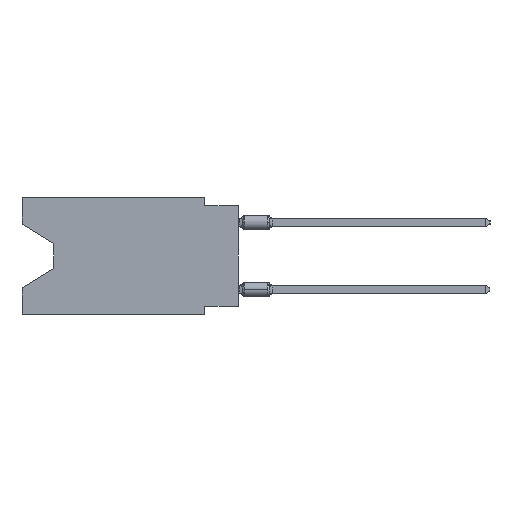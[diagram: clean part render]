
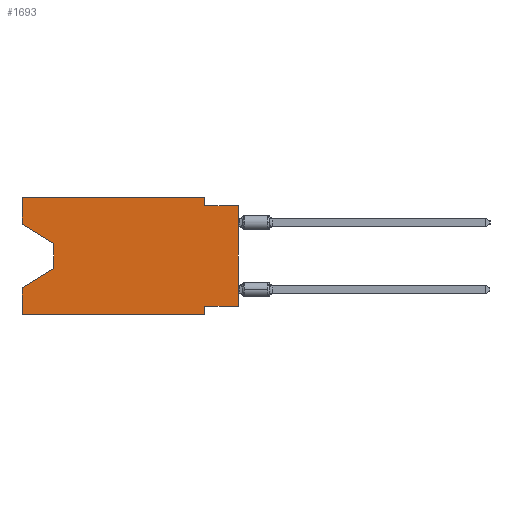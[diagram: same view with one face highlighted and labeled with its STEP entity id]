
A CAD part, left-side view. The second image highlights one B-rep face of the part: STEP entity #1693.
In plain terms, the highlighted planar face has unit normal (-1, 0, 0).
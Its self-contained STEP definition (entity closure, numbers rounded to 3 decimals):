
#61 = CARTESIAN_POINT ( 'NONE',  ( 0., 16.383, -2.038 ) ) ;
#405 = EDGE_CURVE ( 'NONE', #11321, #2770, #20405, .T. ) ;
#503 = CARTESIAN_POINT ( 'NONE',  ( 0., 16.383, -6.852 ) ) ;
#1020 = LINE ( 'NONE', #27238, #17235 ) ;
#1627 = CARTESIAN_POINT ( 'NONE',  ( 0., 0., -0.635 ) ) ;
#1693 = ADVANCED_FACE ( 'NONE', ( #6547 ), #28965, .F. ) ;
#1773 = VECTOR ( 'NONE', #10574, 1000. ) ;
#1826 = DIRECTION ( 'NONE',  ( 0., -1., 0. ) ) ;
#2639 = VECTOR ( 'NONE', #15051, 1000. ) ;
#2770 = VERTEX_POINT ( 'NONE', #3401 ) ;
#2835 = VERTEX_POINT ( 'NONE', #14251 ) ;
#3376 = DIRECTION ( 'NONE',  ( 0., 1., 0. ) ) ;
#3401 = CARTESIAN_POINT ( 'NONE',  ( 0., 2.54, 0. ) ) ;
#3707 = DIRECTION ( 'NONE',  ( 0., 0., -1. ) ) ;
#4141 = VERTEX_POINT ( 'NONE', #28311 ) ;
#4184 = VECTOR ( 'NONE', #5566, 1000. ) ;
#4246 = DIRECTION ( 'NONE',  ( 0., 0., -1. ) ) ;
#4360 = ORIENTED_EDGE ( 'NONE', *, *, #12517, .F. ) ;
#4763 = ORIENTED_EDGE ( 'NONE', *, *, #11720, .T. ) ;
#4791 = CARTESIAN_POINT ( 'NONE',  ( 0., 2.54, -0.635 ) ) ;
#5427 = LINE ( 'NONE', #23144, #12451 ) ;
#5566 = DIRECTION ( 'NONE',  ( 0., 0.855, -0.519 ) ) ;
#5591 = LINE ( 'NONE', #23448, #18573 ) ;
#5696 = CARTESIAN_POINT ( 'NONE',  ( 0., 0., 0. ) ) ;
#6420 = CARTESIAN_POINT ( 'NONE',  ( 0., 2.54, 0. ) ) ;
#6547 = FACE_OUTER_BOUND ( 'NONE', #22709, .T. ) ;
#6698 = CARTESIAN_POINT ( 'NONE',  ( 0., 13.97, -3.505 ) ) ;
#6756 = EDGE_CURVE ( 'NONE', #17908, #6912, #1020, .T. ) ;
#6912 = VERTEX_POINT ( 'NONE', #10834 ) ;
#6955 = LINE ( 'NONE', #27174, #19351 ) ;
#7244 = VERTEX_POINT ( 'NONE', #10662 ) ;
#7461 = VERTEX_POINT ( 'NONE', #11942 ) ;
#8135 = DIRECTION ( 'NONE',  ( 0., 0., -1. ) ) ;
#8440 = ORIENTED_EDGE ( 'NONE', *, *, #9768, .T. ) ;
#8973 = CARTESIAN_POINT ( 'NONE',  ( 0., 16.383, -8.89 ) ) ;
#8974 = EDGE_CURVE ( 'NONE', #4141, #6912, #19122, .T. ) ;
#9768 = EDGE_CURVE ( 'NONE', #11757, #28223, #16980, .T. ) ;
#10574 = DIRECTION ( 'NONE',  ( 0., -1., 0. ) ) ;
#10613 = VERTEX_POINT ( 'NONE', #12658 ) ;
#10662 = CARTESIAN_POINT ( 'NONE',  ( 0., 16.383, -2.038 ) ) ;
#10834 = CARTESIAN_POINT ( 'NONE',  ( 0., 2.54, -8.89 ) ) ;
#10908 = ORIENTED_EDGE ( 'NONE', *, *, #14576, .F. ) ;
#11321 = VERTEX_POINT ( 'NONE', #13165 ) ;
#11524 = ORIENTED_EDGE ( 'NONE', *, *, #17257, .F. ) ;
#11616 = ORIENTED_EDGE ( 'NONE', *, *, #8974, .T. ) ;
#11720 = EDGE_CURVE ( 'NONE', #7244, #2835, #19992, .T. ) ;
#11757 = VERTEX_POINT ( 'NONE', #22618 ) ;
#11942 = CARTESIAN_POINT ( 'NONE',  ( 0., 0., -8.255 ) ) ;
#12451 = VECTOR ( 'NONE', #27549, 1000. ) ;
#12517 = EDGE_CURVE ( 'NONE', #2770, #27686, #22223, .T. ) ;
#12658 = CARTESIAN_POINT ( 'NONE',  ( 0., 0., -0.635 ) ) ;
#12871 = CARTESIAN_POINT ( 'NONE',  ( 0., 16.383, 0. ) ) ;
#13165 = CARTESIAN_POINT ( 'NONE',  ( 0., 16.383, 0. ) ) ;
#14251 = CARTESIAN_POINT ( 'NONE',  ( 0., 13.97, -3.505 ) ) ;
#14576 = EDGE_CURVE ( 'NONE', #7244, #11321, #5427, .T. ) ;
#14627 = DIRECTION ( 'NONE',  ( 0., 0., 1. ) ) ;
#14801 = VECTOR ( 'NONE', #4246, 1000. ) ;
#15051 = DIRECTION ( 'NONE',  ( 0., -0.855, -0.519 ) ) ;
#15369 = VECTOR ( 'NONE', #24939, 1000. ) ;
#15395 = CARTESIAN_POINT ( 'NONE',  ( 0., 2.54, -8.255 ) ) ;
#15619 = DIRECTION ( 'NONE',  ( 1., 0., 0. ) ) ;
#16201 = ORIENTED_EDGE ( 'NONE', *, *, #6756, .F. ) ;
#16521 = AXIS2_PLACEMENT_3D ( 'NONE', #17820, #15619, #8135 ) ;
#16980 = LINE ( 'NONE', #18873, #4184 ) ;
#17117 = ORIENTED_EDGE ( 'NONE', *, *, #405, .F. ) ;
#17235 = VECTOR ( 'NONE', #25466, 1000. ) ;
#17257 = EDGE_CURVE ( 'NONE', #27686, #10613, #19769, .T. ) ;
#17820 = CARTESIAN_POINT ( 'NONE',  ( 0., 16.383, 0. ) ) ;
#17908 = VERTEX_POINT ( 'NONE', #15395 ) ;
#18573 = VECTOR ( 'NONE', #3376, 1000. ) ;
#18873 = CARTESIAN_POINT ( 'NONE',  ( 0., 13.97, -5.385 ) ) ;
#19122 = LINE ( 'NONE', #8973, #27064 ) ;
#19351 = VECTOR ( 'NONE', #24674, 1000. ) ;
#19550 = VECTOR ( 'NONE', #3707, 1000. ) ;
#19769 = LINE ( 'NONE', #1627, #1773 ) ;
#19992 = LINE ( 'NONE', #61, #2639 ) ;
#20405 = LINE ( 'NONE', #12871, #15369 ) ;
#21037 = ORIENTED_EDGE ( 'NONE', *, *, #23453, .T. ) ;
#21209 = LINE ( 'NONE', #5696, #22520 ) ;
#21337 = EDGE_CURVE ( 'NONE', #4141, #28223, #6955, .T. ) ;
#21554 = ORIENTED_EDGE ( 'NONE', *, *, #25008, .T. ) ;
#21968 = LINE ( 'NONE', #6698, #14801 ) ;
#22223 = LINE ( 'NONE', #6420, #19550 ) ;
#22520 = VECTOR ( 'NONE', #14627, 1000. ) ;
#22618 = CARTESIAN_POINT ( 'NONE',  ( 0., 13.97, -5.385 ) ) ;
#22709 = EDGE_LOOP ( 'NONE', ( #4763, #21037, #8440, #23082, #11616, #16201, #25721, #21554, #11524, #4360, #17117, #10908 ) ) ;
#23082 = ORIENTED_EDGE ( 'NONE', *, *, #21337, .F. ) ;
#23144 = CARTESIAN_POINT ( 'NONE',  ( 0., 16.383, 0. ) ) ;
#23448 = CARTESIAN_POINT ( 'NONE',  ( 0., 0., -8.255 ) ) ;
#23453 = EDGE_CURVE ( 'NONE', #2835, #11757, #21968, .T. ) ;
#24674 = DIRECTION ( 'NONE',  ( 0., 0., 1. ) ) ;
#24939 = DIRECTION ( 'NONE',  ( 0., -1., 0. ) ) ;
#25008 = EDGE_CURVE ( 'NONE', #7461, #10613, #21209, .T. ) ;
#25466 = DIRECTION ( 'NONE',  ( 0., 0., -1. ) ) ;
#25721 = ORIENTED_EDGE ( 'NONE', *, *, #25955, .F. ) ;
#25955 = EDGE_CURVE ( 'NONE', #7461, #17908, #5591, .T. ) ;
#27064 = VECTOR ( 'NONE', #1826, 1000. ) ;
#27174 = CARTESIAN_POINT ( 'NONE',  ( 0., 16.383, 0. ) ) ;
#27238 = CARTESIAN_POINT ( 'NONE',  ( 0., 2.54, -8.89 ) ) ;
#27549 = DIRECTION ( 'NONE',  ( 0., 0., 1. ) ) ;
#27686 = VERTEX_POINT ( 'NONE', #4791 ) ;
#28223 = VERTEX_POINT ( 'NONE', #503 ) ;
#28311 = CARTESIAN_POINT ( 'NONE',  ( 0., 16.383, -8.89 ) ) ;
#28965 = PLANE ( 'NONE',  #16521 ) ;
